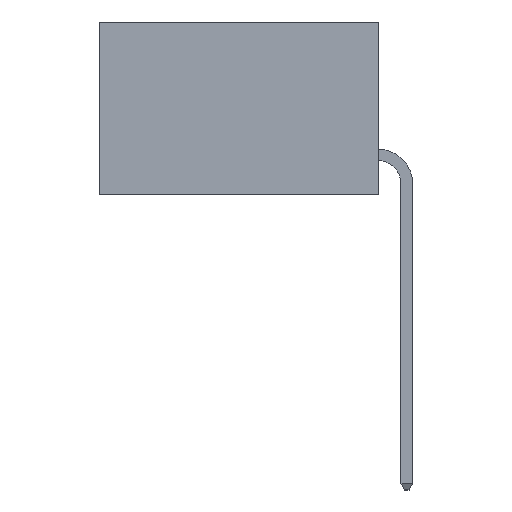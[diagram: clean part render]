
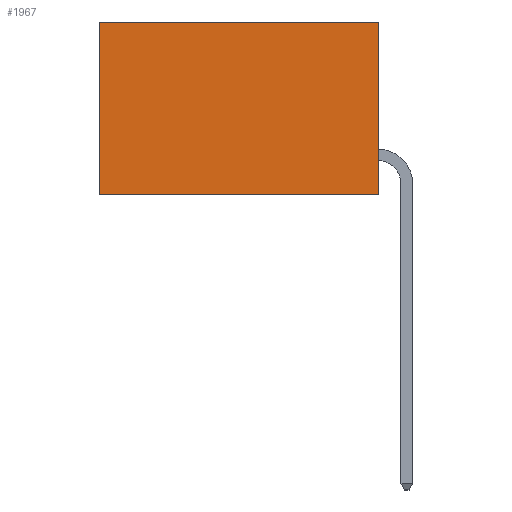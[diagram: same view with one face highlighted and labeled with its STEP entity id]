
A CAD part, left-side view. The second image highlights one B-rep face of the part: STEP entity #1967.
In plain terms, the highlighted planar face has unit normal (-1, 0, 0).
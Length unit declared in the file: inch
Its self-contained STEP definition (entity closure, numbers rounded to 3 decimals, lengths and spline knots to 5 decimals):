
#558 = EDGE_CURVE ( 'NONE', #7119, #5639, #4282, .T. ) ;
#1134 = EDGE_LOOP ( 'NONE', ( #8805, #10661, #10575, #9157 ) ) ;
#1473 = CARTESIAN_POINT ( 'NONE',  ( 0.2615, 0., -0.37 ) ) ;
#1967 = ADVANCED_FACE ( 'NONE', ( #3565 ), #5433, .F. ) ;
#2060 = VERTEX_POINT ( 'NONE', #10672 ) ;
#2113 = EDGE_CURVE ( 'NONE', #2466, #2060, #10355, .T. ) ;
#2466 = VERTEX_POINT ( 'NONE', #4588 ) ;
#2987 = LINE ( 'NONE', #3593, #9151 ) ;
#3431 = CARTESIAN_POINT ( 'NONE',  ( 0.2615, 0., -0.37 ) ) ;
#3451 = DIRECTION ( 'NONE',  ( 0., 1., 0. ) ) ;
#3565 = FACE_OUTER_BOUND ( 'NONE', #1134, .T. ) ;
#3593 = CARTESIAN_POINT ( 'NONE',  ( 0.2615, 0., -0.37 ) ) ;
#3783 = EDGE_CURVE ( 'NONE', #2060, #5639, #2987, .T. ) ;
#4282 = LINE ( 'NONE', #7135, #6520 ) ;
#4588 = CARTESIAN_POINT ( 'NONE',  ( 0.2615, 0., 0. ) ) ;
#4861 = DIRECTION ( 'NONE',  ( 0., 1., 0. ) ) ;
#4892 = LINE ( 'NONE', #8923, #8981 ) ;
#5433 = PLANE ( 'NONE',  #6987 ) ;
#5639 = VERTEX_POINT ( 'NONE', #6986 ) ;
#5872 = EDGE_CURVE ( 'NONE', #2466, #7119, #4892, .T. ) ;
#6520 = VECTOR ( 'NONE', #10342, 39.37008 ) ;
#6986 = CARTESIAN_POINT ( 'NONE',  ( 0.2615, 0.6, -0.37 ) ) ;
#6987 = AXIS2_PLACEMENT_3D ( 'NONE', #1473, #9138, #7188 ) ;
#7119 = VERTEX_POINT ( 'NONE', #8438 ) ;
#7135 = CARTESIAN_POINT ( 'NONE',  ( 0.2615, 0.6, -0.37 ) ) ;
#7188 = DIRECTION ( 'NONE',  ( 0., 0., -1. ) ) ;
#8397 = VECTOR ( 'NONE', #10786, 39.37008 ) ;
#8438 = CARTESIAN_POINT ( 'NONE',  ( 0.2615, 0.6, 0. ) ) ;
#8805 = ORIENTED_EDGE ( 'NONE', *, *, #558, .T. ) ;
#8923 = CARTESIAN_POINT ( 'NONE',  ( 0.2615, 0., 0. ) ) ;
#8981 = VECTOR ( 'NONE', #4861, 39.37008 ) ;
#9138 = DIRECTION ( 'NONE',  ( 1., 0., 0. ) ) ;
#9151 = VECTOR ( 'NONE', #3451, 39.37008 ) ;
#9157 = ORIENTED_EDGE ( 'NONE', *, *, #5872, .T. ) ;
#10342 = DIRECTION ( 'NONE',  ( 0., 0., -1. ) ) ;
#10355 = LINE ( 'NONE', #3431, #8397 ) ;
#10575 = ORIENTED_EDGE ( 'NONE', *, *, #2113, .F. ) ;
#10661 = ORIENTED_EDGE ( 'NONE', *, *, #3783, .F. ) ;
#10672 = CARTESIAN_POINT ( 'NONE',  ( 0.2615, 0., -0.37 ) ) ;
#10786 = DIRECTION ( 'NONE',  ( 0., 0., -1. ) ) ;
